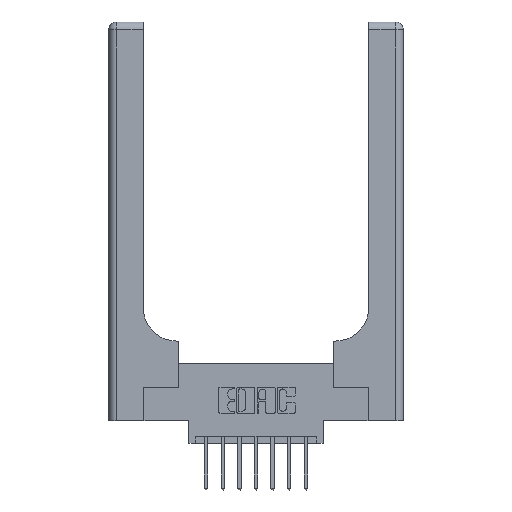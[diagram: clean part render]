
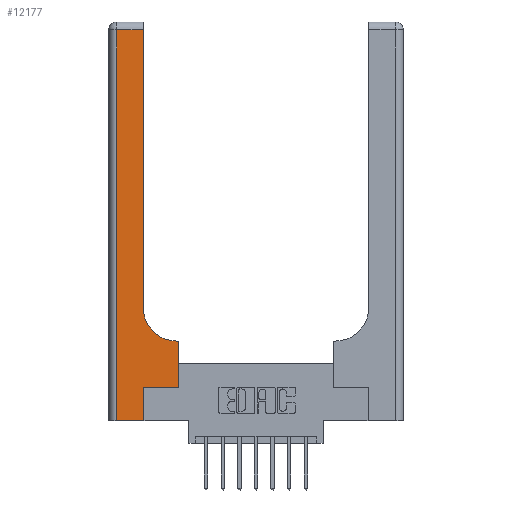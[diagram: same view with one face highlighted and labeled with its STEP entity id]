
A CAD part, top view. The second image highlights one B-rep face of the part: STEP entity #12177.
In plain terms, the highlighted planar face has unit normal (0, 0, 1).
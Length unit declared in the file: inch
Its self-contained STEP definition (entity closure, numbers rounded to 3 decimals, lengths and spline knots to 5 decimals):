
#124 = CARTESIAN_POINT ( 'NONE',  ( 0.528, 0.25, 0.37 ) ) ;
#742 = DIRECTION ( 'NONE',  ( 0., 1., 0. ) ) ;
#1562 = EDGE_CURVE ( 'NONE', #9122, #1946, #11609, .T. ) ;
#1684 = VECTOR ( 'NONE', #2326, 39.37008 ) ;
#1765 = EDGE_CURVE ( 'NONE', #1946, #12378, #13637, .T. ) ;
#1772 = DIRECTION ( 'NONE',  ( -1., 0., 0. ) ) ;
#1946 = VERTEX_POINT ( 'NONE', #5717 ) ;
#2086 = DIRECTION ( 'NONE',  ( 0., -1., 0. ) ) ;
#2178 = VECTOR ( 'NONE', #2086, 39.37008 ) ;
#2211 = DIRECTION ( 'NONE',  ( 1., 0., 0. ) ) ;
#2326 = DIRECTION ( 'NONE',  ( -1., 0., 0. ) ) ;
#2557 = EDGE_CURVE ( 'NONE', #12380, #9122, #11109, .T. ) ;
#2596 = CARTESIAN_POINT ( 'NONE',  ( 0.26, 2.94, 0.37 ) ) ;
#2793 = EDGE_CURVE ( 'NONE', #12022, #3035, #7333, .T. ) ;
#3035 = VERTEX_POINT ( 'NONE', #5788 ) ;
#3359 = CARTESIAN_POINT ( 'NONE',  ( 0.06, 0., 0.37 ) ) ;
#3366 = ORIENTED_EDGE ( 'NONE', *, *, #9674, .T. ) ;
#3518 = EDGE_CURVE ( 'NONE', #12378, #12022, #10217, .T. ) ;
#4054 = LINE ( 'NONE', #10986, #14647 ) ;
#4468 = DIRECTION ( 'NONE',  ( 1., 0., 0. ) ) ;
#4886 = CARTESIAN_POINT ( 'NONE',  ( 0.51, 0.85, 0.37 ) ) ;
#5410 = CARTESIAN_POINT ( 'NONE',  ( 0.06, 3., 0.37 ) ) ;
#5479 = ORIENTED_EDGE ( 'NONE', *, *, #1765, .T. ) ;
#5586 = VERTEX_POINT ( 'NONE', #13981 ) ;
#5596 = VECTOR ( 'NONE', #742, 39.37008 ) ;
#5665 = VECTOR ( 'NONE', #7112, 39.37008 ) ;
#5717 = CARTESIAN_POINT ( 'NONE',  ( 0.06, 2.94, 0.37 ) ) ;
#5788 = CARTESIAN_POINT ( 'NONE',  ( 0.265, 0.25, 0.37 ) ) ;
#5961 = CARTESIAN_POINT ( 'NONE',  ( 0., 2.94, 0.37 ) ) ;
#6265 = CARTESIAN_POINT ( 'NONE',  ( 0.265, 0., 0.37 ) ) ;
#6941 = CARTESIAN_POINT ( 'NONE',  ( 0.26, 0.85, 0.37 ) ) ;
#7019 = ORIENTED_EDGE ( 'NONE', *, *, #2793, .T. ) ;
#7112 = DIRECTION ( 'NONE',  ( 0., 1., 0. ) ) ;
#7133 = CARTESIAN_POINT ( 'NONE',  ( 0.528, 0.25, 0.37 ) ) ;
#7197 = VECTOR ( 'NONE', #2211, 39.37008 ) ;
#7333 = LINE ( 'NONE', #6265, #13495 ) ;
#7345 = VECTOR ( 'NONE', #4468, 39.37008 ) ;
#8007 = CARTESIAN_POINT ( 'NONE',  ( 0., 0., 0.37 ) ) ;
#8103 = EDGE_CURVE ( 'NONE', #3035, #9322, #12604, .T. ) ;
#8279 = ORIENTED_EDGE ( 'NONE', *, *, #3518, .T. ) ;
#8420 = DIRECTION ( 'NONE',  ( 0., 0., -1. ) ) ;
#8636 = PLANE ( 'NONE',  #12961 ) ;
#8805 = AXIS2_PLACEMENT_3D ( 'NONE', #4886, #8420, #10775 ) ;
#9122 = VERTEX_POINT ( 'NONE', #2596 ) ;
#9289 = CARTESIAN_POINT ( 'NONE',  ( 0.51, 0.6, 0.37 ) ) ;
#9322 = VERTEX_POINT ( 'NONE', #7133 ) ;
#9423 = CARTESIAN_POINT ( 'NONE',  ( 0.265, 0.25, 0.37 ) ) ;
#9674 = EDGE_CURVE ( 'NONE', #9322, #5586, #10557, .T. ) ;
#9772 = CARTESIAN_POINT ( 'NONE',  ( 0., 3., 0.37 ) ) ;
#9923 = DIRECTION ( 'NONE',  ( -1., 0., 0. ) ) ;
#10217 = LINE ( 'NONE', #8007, #7197 ) ;
#10290 = ORIENTED_EDGE ( 'NONE', *, *, #2557, .T. ) ;
#10557 = LINE ( 'NONE', #124, #5665 ) ;
#10775 = DIRECTION ( 'NONE',  ( 1., 0., 0. ) ) ;
#10809 = EDGE_LOOP ( 'NONE', ( #10290, #14789, #5479, #8279, #7019, #14181, #3366, #12131, #12545 ) ) ;
#10986 = CARTESIAN_POINT ( 'NONE',  ( 0.26, 0.6, 0.37 ) ) ;
#11109 = LINE ( 'NONE', #12314, #5596 ) ;
#11142 = DIRECTION ( 'NONE',  ( 0., 1., 0. ) ) ;
#11609 = LINE ( 'NONE', #5961, #1684 ) ;
#11763 = CARTESIAN_POINT ( 'NONE',  ( 0.265, 0., 0.37 ) ) ;
#12022 = VERTEX_POINT ( 'NONE', #11763 ) ;
#12131 = ORIENTED_EDGE ( 'NONE', *, *, #12171, .T. ) ;
#12171 = EDGE_CURVE ( 'NONE', #5586, #12861, #4054, .T. ) ;
#12177 = ADVANCED_FACE ( 'NONE', ( #13262 ), #8636, .F. ) ;
#12314 = CARTESIAN_POINT ( 'NONE',  ( 0.26, 3., 0.37 ) ) ;
#12378 = VERTEX_POINT ( 'NONE', #3359 ) ;
#12380 = VERTEX_POINT ( 'NONE', #6941 ) ;
#12545 = ORIENTED_EDGE ( 'NONE', *, *, #15008, .T. ) ;
#12604 = LINE ( 'NONE', #9423, #7345 ) ;
#12861 = VERTEX_POINT ( 'NONE', #9289 ) ;
#12961 = AXIS2_PLACEMENT_3D ( 'NONE', #9772, #13334, #9923 ) ;
#13262 = FACE_OUTER_BOUND ( 'NONE', #10809, .T. ) ;
#13334 = DIRECTION ( 'NONE',  ( 0., 0., -1. ) ) ;
#13495 = VECTOR ( 'NONE', #11142, 39.37008 ) ;
#13637 = LINE ( 'NONE', #5410, #2178 ) ;
#13981 = CARTESIAN_POINT ( 'NONE',  ( 0.528, 0.6, 0.37 ) ) ;
#14181 = ORIENTED_EDGE ( 'NONE', *, *, #8103, .T. ) ;
#14377 = CIRCLE ( 'NONE', #8805, 0.25 ) ;
#14647 = VECTOR ( 'NONE', #1772, 39.37008 ) ;
#14789 = ORIENTED_EDGE ( 'NONE', *, *, #1562, .T. ) ;
#15008 = EDGE_CURVE ( 'NONE', #12861, #12380, #14377, .T. ) ;
